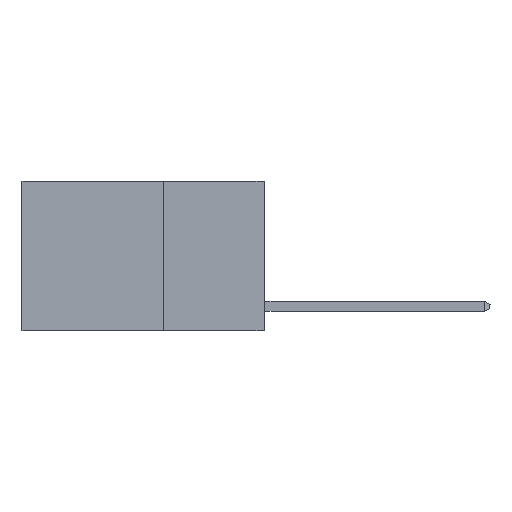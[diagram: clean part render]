
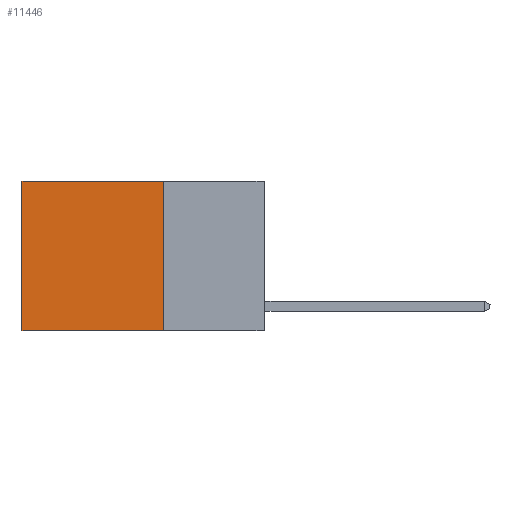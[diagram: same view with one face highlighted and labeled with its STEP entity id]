
A CAD part, left-side view. The second image highlights one B-rep face of the part: STEP entity #11446.
In plain terms, the highlighted planar face has unit normal (-1, 0, 0).
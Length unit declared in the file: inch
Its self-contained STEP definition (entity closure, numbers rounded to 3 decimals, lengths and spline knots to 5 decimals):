
#92 = ORIENTED_EDGE ( 'NONE', *, *, #6314, .T. ) ;
#325 = DIRECTION ( 'NONE',  ( 1., 0., 0. ) ) ;
#1439 = FACE_OUTER_BOUND ( 'NONE', #9136, .T. ) ;
#1664 = VERTEX_POINT ( 'NONE', #6609 ) ;
#1933 = EDGE_CURVE ( 'NONE', #1664, #10003, #5398, .T. ) ;
#2093 = LINE ( 'NONE', #3877, #10302 ) ;
#2374 = DIRECTION ( 'NONE',  ( 0., 0., -1. ) ) ;
#2542 = LINE ( 'NONE', #8330, #8653 ) ;
#2770 = CARTESIAN_POINT ( 'NONE',  ( 0.2625, 0.25, -0.37 ) ) ;
#2932 = VECTOR ( 'NONE', #11911, 39.37008 ) ;
#3314 = EDGE_CURVE ( 'NONE', #1664, #8435, #2093, .T. ) ;
#3494 = AXIS2_PLACEMENT_3D ( 'NONE', #6417, #325, #5217 ) ;
#3659 = ORIENTED_EDGE ( 'NONE', *, *, #3314, .T. ) ;
#3877 = CARTESIAN_POINT ( 'NONE',  ( 0.2625, 0.25, 0. ) ) ;
#4261 = EDGE_CURVE ( 'NONE', #10003, #9332, #6892, .T. ) ;
#4327 = DIRECTION ( 'NONE',  ( 0., 0., -1. ) ) ;
#4431 = CARTESIAN_POINT ( 'NONE',  ( 0.2625, 0.25, 0. ) ) ;
#5217 = DIRECTION ( 'NONE',  ( 0., 0., -1. ) ) ;
#5398 = LINE ( 'NONE', #4431, #7178 ) ;
#6038 = CARTESIAN_POINT ( 'NONE',  ( 0.2625, 0.6, 0. ) ) ;
#6296 = PLANE ( 'NONE',  #3494 ) ;
#6314 = EDGE_CURVE ( 'NONE', #8435, #9332, #2542, .T. ) ;
#6417 = CARTESIAN_POINT ( 'NONE',  ( 0.2625, 0.25, 0. ) ) ;
#6524 = ORIENTED_EDGE ( 'NONE', *, *, #4261, .F. ) ;
#6609 = CARTESIAN_POINT ( 'NONE',  ( 0.2625, 0.25, 0. ) ) ;
#6892 = LINE ( 'NONE', #2770, #2932 ) ;
#7178 = VECTOR ( 'NONE', #4327, 39.37008 ) ;
#8312 = CARTESIAN_POINT ( 'NONE',  ( 0.2625, 0.6, -0.37 ) ) ;
#8330 = CARTESIAN_POINT ( 'NONE',  ( 0.2625, 0.6, 0. ) ) ;
#8435 = VERTEX_POINT ( 'NONE', #6038 ) ;
#8653 = VECTOR ( 'NONE', #2374, 39.37008 ) ;
#8971 = DIRECTION ( 'NONE',  ( 0., 1., 0. ) ) ;
#9136 = EDGE_LOOP ( 'NONE', ( #92, #6524, #9545, #3659 ) ) ;
#9332 = VERTEX_POINT ( 'NONE', #8312 ) ;
#9545 = ORIENTED_EDGE ( 'NONE', *, *, #1933, .F. ) ;
#9576 = CARTESIAN_POINT ( 'NONE',  ( 0.2625, 0.25, -0.37 ) ) ;
#10003 = VERTEX_POINT ( 'NONE', #9576 ) ;
#10302 = VECTOR ( 'NONE', #8971, 39.37008 ) ;
#11446 = ADVANCED_FACE ( 'NONE', ( #1439 ), #6296, .F. ) ;
#11911 = DIRECTION ( 'NONE',  ( 0., 1., 0. ) ) ;
